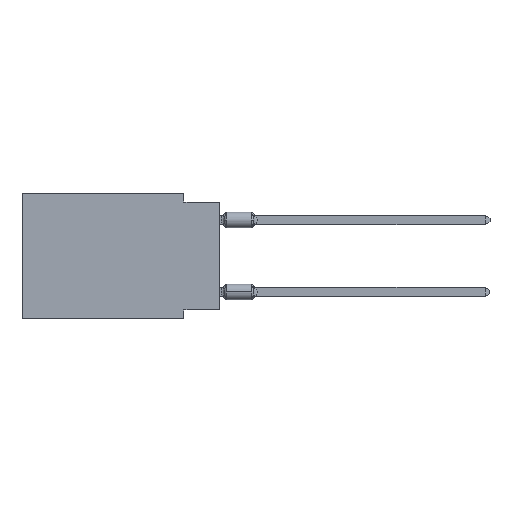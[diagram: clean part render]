
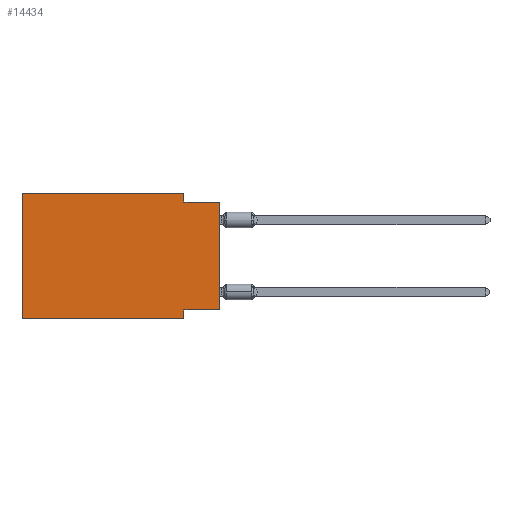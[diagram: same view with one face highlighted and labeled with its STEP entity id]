
A CAD part, left-side view. The second image highlights one B-rep face of the part: STEP entity #14434.
In plain terms, the highlighted planar face has unit normal (-1, 0, 0).
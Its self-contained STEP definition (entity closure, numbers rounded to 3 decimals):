
#612 = EDGE_CURVE ( 'NONE', #1995, #2593, #14900, .T. ) ;
#671 = VERTEX_POINT ( 'NONE', #19172 ) ;
#812 = VECTOR ( 'NONE', #11148, 1000. ) ;
#895 = DIRECTION ( 'NONE',  ( 0., -1., 0. ) ) ;
#1057 = DIRECTION ( 'NONE',  ( 0., 0., 1. ) ) ;
#1063 = EDGE_CURVE ( 'NONE', #12840, #18130, #5733, .T. ) ;
#1754 = CARTESIAN_POINT ( 'NONE',  ( 0., 2.54, -8.255 ) ) ;
#1825 = VECTOR ( 'NONE', #1057, 1000. ) ;
#1995 = VERTEX_POINT ( 'NONE', #7185 ) ;
#2173 = AXIS2_PLACEMENT_3D ( 'NONE', #9315, #16681, #9024 ) ;
#2593 = VERTEX_POINT ( 'NONE', #12476 ) ;
#2736 = DIRECTION ( 'NONE',  ( 0., 1., 0. ) ) ;
#3103 = CARTESIAN_POINT ( 'NONE',  ( 0., 13.97, -8.89 ) ) ;
#3186 = ORIENTED_EDGE ( 'NONE', *, *, #1063, .T. ) ;
#3730 = VECTOR ( 'NONE', #14363, 1000. ) ;
#4052 = ORIENTED_EDGE ( 'NONE', *, *, #9328, .F. ) ;
#4178 = LINE ( 'NONE', #10320, #18206 ) ;
#4301 = VECTOR ( 'NONE', #13619, 1000. ) ;
#4313 = LINE ( 'NONE', #7397, #4999 ) ;
#4999 = VECTOR ( 'NONE', #2736, 1000. ) ;
#5220 = CARTESIAN_POINT ( 'NONE',  ( 0., 2.54, 0. ) ) ;
#5457 = ORIENTED_EDGE ( 'NONE', *, *, #13542, .F. ) ;
#5733 = LINE ( 'NONE', #8799, #1825 ) ;
#6941 = EDGE_CURVE ( 'NONE', #671, #18130, #12643, .T. ) ;
#7185 = CARTESIAN_POINT ( 'NONE',  ( 0., 13.97, 0. ) ) ;
#7232 = LINE ( 'NONE', #16646, #15156 ) ;
#7283 = EDGE_CURVE ( 'NONE', #17095, #13616, #18184, .T. ) ;
#7397 = CARTESIAN_POINT ( 'NONE',  ( 0., 0., -8.255 ) ) ;
#7558 = FACE_OUTER_BOUND ( 'NONE', #11337, .T. ) ;
#8799 = CARTESIAN_POINT ( 'NONE',  ( 0., 0., 0. ) ) ;
#9024 = DIRECTION ( 'NONE',  ( 0., 0., -1. ) ) ;
#9315 = CARTESIAN_POINT ( 'NONE',  ( 0., 13.97, 0. ) ) ;
#9328 = EDGE_CURVE ( 'NONE', #17095, #1995, #7232, .T. ) ;
#9343 = ORIENTED_EDGE ( 'NONE', *, *, #7283, .T. ) ;
#9956 = EDGE_CURVE ( 'NONE', #13279, #13616, #4178, .T. ) ;
#10217 = DIRECTION ( 'NONE',  ( 0., 0., -1. ) ) ;
#10289 = DIRECTION ( 'NONE',  ( 0., 0., 1. ) ) ;
#10320 = CARTESIAN_POINT ( 'NONE',  ( 0., 2.54, -8.89 ) ) ;
#10871 = ORIENTED_EDGE ( 'NONE', *, *, #612, .F. ) ;
#11148 = DIRECTION ( 'NONE',  ( 0., -1., 0. ) ) ;
#11303 = CARTESIAN_POINT ( 'NONE',  ( 0., 0., -0.635 ) ) ;
#11337 = EDGE_LOOP ( 'NONE', ( #3186, #14030, #13522, #10871, #4052, #9343, #18907, #5457 ) ) ;
#12367 = CARTESIAN_POINT ( 'NONE',  ( 0., 2.54, -8.89 ) ) ;
#12476 = CARTESIAN_POINT ( 'NONE',  ( 0., 2.54, 0. ) ) ;
#12643 = LINE ( 'NONE', #18714, #812 ) ;
#12840 = VERTEX_POINT ( 'NONE', #16800 ) ;
#13279 = VERTEX_POINT ( 'NONE', #1754 ) ;
#13385 = EDGE_CURVE ( 'NONE', #2593, #671, #14175, .T. ) ;
#13522 = ORIENTED_EDGE ( 'NONE', *, *, #13385, .F. ) ;
#13542 = EDGE_CURVE ( 'NONE', #12840, #13279, #4313, .T. ) ;
#13616 = VERTEX_POINT ( 'NONE', #12367 ) ;
#13619 = DIRECTION ( 'NONE',  ( 0., -1., 0. ) ) ;
#14030 = ORIENTED_EDGE ( 'NONE', *, *, #6941, .F. ) ;
#14175 = LINE ( 'NONE', #5220, #3730 ) ;
#14363 = DIRECTION ( 'NONE',  ( 0., 0., -1. ) ) ;
#14434 = ADVANCED_FACE ( 'NONE', ( #7558 ), #18080, .F. ) ;
#14900 = LINE ( 'NONE', #17678, #18742 ) ;
#15156 = VECTOR ( 'NONE', #10289, 1000. ) ;
#16646 = CARTESIAN_POINT ( 'NONE',  ( 0., 13.97, 0. ) ) ;
#16681 = DIRECTION ( 'NONE',  ( 1., 0., 0. ) ) ;
#16800 = CARTESIAN_POINT ( 'NONE',  ( 0., 0., -8.255 ) ) ;
#16935 = CARTESIAN_POINT ( 'NONE',  ( 0., 13.97, -8.89 ) ) ;
#17095 = VERTEX_POINT ( 'NONE', #16935 ) ;
#17678 = CARTESIAN_POINT ( 'NONE',  ( 0., 13.97, 0. ) ) ;
#18080 = PLANE ( 'NONE',  #2173 ) ;
#18130 = VERTEX_POINT ( 'NONE', #11303 ) ;
#18184 = LINE ( 'NONE', #3103, #4301 ) ;
#18206 = VECTOR ( 'NONE', #10217, 1000. ) ;
#18714 = CARTESIAN_POINT ( 'NONE',  ( 0., 0., -0.635 ) ) ;
#18742 = VECTOR ( 'NONE', #895, 1000. ) ;
#18907 = ORIENTED_EDGE ( 'NONE', *, *, #9956, .F. ) ;
#19172 = CARTESIAN_POINT ( 'NONE',  ( 0., 2.54, -0.635 ) ) ;
